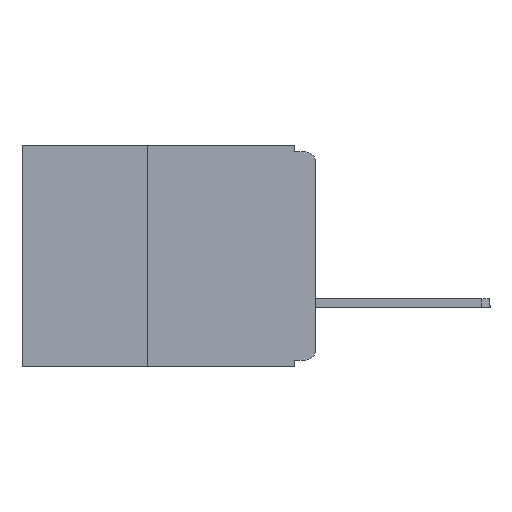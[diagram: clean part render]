
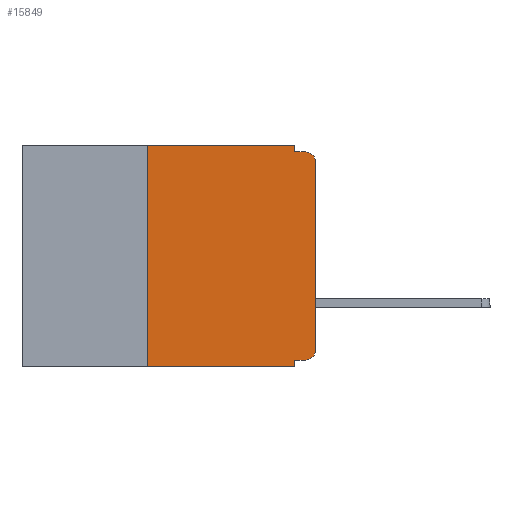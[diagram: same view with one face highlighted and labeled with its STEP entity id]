
A CAD part, left-side view. The second image highlights one B-rep face of the part: STEP entity #15849.
In plain terms, the highlighted planar face has unit normal (-1, 0, 0).
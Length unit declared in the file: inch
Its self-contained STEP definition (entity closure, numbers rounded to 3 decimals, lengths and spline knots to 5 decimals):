
#66 = DIRECTION ( 'NONE',  ( 0., -1., 0. ) ) ;
#398 = VERTEX_POINT ( 'NONE', #6209 ) ;
#481 = ORIENTED_EDGE ( 'NONE', *, *, #9868, .F. ) ;
#497 = CARTESIAN_POINT ( 'NONE',  ( 0., 0.031, -0.33 ) ) ;
#763 = VERTEX_POINT ( 'NONE', #16067 ) ;
#864 = VERTEX_POINT ( 'NONE', #1118 ) ;
#1118 = CARTESIAN_POINT ( 'NONE',  ( 0., 0.25, -0.33 ) ) ;
#1212 = CIRCLE ( 'NONE', #5402, 0.015 ) ;
#1240 = VECTOR ( 'NONE', #4410, 39.37008 ) ;
#1296 = FACE_OUTER_BOUND ( 'NONE', #16125, .T. ) ;
#1374 = EDGE_CURVE ( 'NONE', #15791, #12841, #13260, .T. ) ;
#1421 = AXIS2_PLACEMENT_3D ( 'NONE', #1442, #10555, #2855 ) ;
#1430 = EDGE_CURVE ( 'NONE', #864, #16133, #8579, .T. ) ;
#1442 = CARTESIAN_POINT ( 'NONE',  ( 0., 0.015, -0.305 ) ) ;
#1517 = EDGE_CURVE ( 'NONE', #864, #12063, #13790, .T. ) ;
#1592 = EDGE_CURVE ( 'NONE', #398, #12063, #15731, .T. ) ;
#1949 = VECTOR ( 'NONE', #4954, 39.37008 ) ;
#1961 = EDGE_CURVE ( 'NONE', #16133, #15791, #3544, .T. ) ;
#2298 = CIRCLE ( 'NONE', #1421, 0.015 ) ;
#2405 = CARTESIAN_POINT ( 'NONE',  ( 0., 0.437, 0. ) ) ;
#2565 = DIRECTION ( 'NONE',  ( 0., -1., 0. ) ) ;
#2602 = VECTOR ( 'NONE', #11193, 39.37008 ) ;
#2855 = DIRECTION ( 'NONE',  ( 0., 0., -1. ) ) ;
#3038 = ORIENTED_EDGE ( 'NONE', *, *, #10519, .T. ) ;
#3155 = VECTOR ( 'NONE', #2565, 39.37008 ) ;
#3258 = ORIENTED_EDGE ( 'NONE', *, *, #1517, .T. ) ;
#3544 = LINE ( 'NONE', #2405, #3155 ) ;
#3656 = ORIENTED_EDGE ( 'NONE', *, *, #1592, .F. ) ;
#4275 = ORIENTED_EDGE ( 'NONE', *, *, #9363, .F. ) ;
#4373 = CARTESIAN_POINT ( 'NONE',  ( 0., 0.031, 0. ) ) ;
#4410 = DIRECTION ( 'NONE',  ( 0., -1., 0. ) ) ;
#4485 = CARTESIAN_POINT ( 'NONE',  ( 0., 0.437, 0. ) ) ;
#4859 = LINE ( 'NONE', #8299, #1240 ) ;
#4954 = DIRECTION ( 'NONE',  ( 0., 0., 1. ) ) ;
#5307 = ORIENTED_EDGE ( 'NONE', *, *, #8946, .T. ) ;
#5323 = CARTESIAN_POINT ( 'NONE',  ( 0., 0., -0.32 ) ) ;
#5402 = AXIS2_PLACEMENT_3D ( 'NONE', #14794, #7637, #15915 ) ;
#5617 = AXIS2_PLACEMENT_3D ( 'NONE', #4485, #7090, #5811 ) ;
#5811 = DIRECTION ( 'NONE',  ( 0., 0., -1. ) ) ;
#6209 = CARTESIAN_POINT ( 'NONE',  ( 0., 0.031, -0.32 ) ) ;
#6341 = CARTESIAN_POINT ( 'NONE',  ( 0., 0., 0. ) ) ;
#6373 = ORIENTED_EDGE ( 'NONE', *, *, #1430, .F. ) ;
#7090 = DIRECTION ( 'NONE',  ( 1., 0., 0. ) ) ;
#7151 = VECTOR ( 'NONE', #13628, 39.37008 ) ;
#7637 = DIRECTION ( 'NONE',  ( -1., 0., 0. ) ) ;
#7971 = ORIENTED_EDGE ( 'NONE', *, *, #10731, .T. ) ;
#8163 = ORIENTED_EDGE ( 'NONE', *, *, #1374, .F. ) ;
#8299 = CARTESIAN_POINT ( 'NONE',  ( 0., 0., -0.01 ) ) ;
#8379 = VERTEX_POINT ( 'NONE', #12736 ) ;
#8503 = CARTESIAN_POINT ( 'NONE',  ( 0., 0.031, 0. ) ) ;
#8579 = LINE ( 'NONE', #13566, #1949 ) ;
#8634 = VERTEX_POINT ( 'NONE', #14252 ) ;
#8934 = ORIENTED_EDGE ( 'NONE', *, *, #1961, .F. ) ;
#8946 = EDGE_CURVE ( 'NONE', #8379, #9109, #10443, .T. ) ;
#9079 = LINE ( 'NONE', #5323, #15348 ) ;
#9109 = VERTEX_POINT ( 'NONE', #11525 ) ;
#9363 = EDGE_CURVE ( 'NONE', #12841, #8634, #4859, .T. ) ;
#9505 = CARTESIAN_POINT ( 'NONE',  ( 0., 0.437, -0.33 ) ) ;
#9709 = VECTOR ( 'NONE', #10794, 39.37008 ) ;
#9868 = EDGE_CURVE ( 'NONE', #763, #398, #9079, .T. ) ;
#9962 = CARTESIAN_POINT ( 'NONE',  ( 0., 0.031, -0.33 ) ) ;
#10443 = LINE ( 'NONE', #6341, #7151 ) ;
#10519 = EDGE_CURVE ( 'NONE', #9109, #8634, #1212, .T. ) ;
#10555 = DIRECTION ( 'NONE',  ( -1., 0., 0. ) ) ;
#10731 = EDGE_CURVE ( 'NONE', #763, #8379, #2298, .T. ) ;
#10794 = DIRECTION ( 'NONE',  ( 0., 0., -1. ) ) ;
#11193 = DIRECTION ( 'NONE',  ( 0., 0., -1. ) ) ;
#11525 = CARTESIAN_POINT ( 'NONE',  ( 0., 0., -0.025 ) ) ;
#12012 = PLANE ( 'NONE',  #5617 ) ;
#12063 = VERTEX_POINT ( 'NONE', #9962 ) ;
#12316 = CARTESIAN_POINT ( 'NONE',  ( 0., 0.25, 0. ) ) ;
#12736 = CARTESIAN_POINT ( 'NONE',  ( 0., 0., -0.305 ) ) ;
#12841 = VERTEX_POINT ( 'NONE', #13630 ) ;
#13260 = LINE ( 'NONE', #8503, #9709 ) ;
#13429 = VECTOR ( 'NONE', #66, 39.37008 ) ;
#13566 = CARTESIAN_POINT ( 'NONE',  ( 0., 0.25, -0.33 ) ) ;
#13628 = DIRECTION ( 'NONE',  ( 0., 0., 1. ) ) ;
#13630 = CARTESIAN_POINT ( 'NONE',  ( 0., 0.031, -0.01 ) ) ;
#13790 = LINE ( 'NONE', #9505, #13429 ) ;
#13913 = DIRECTION ( 'NONE',  ( 0., 1., 0. ) ) ;
#14252 = CARTESIAN_POINT ( 'NONE',  ( 0., 0.015, -0.01 ) ) ;
#14794 = CARTESIAN_POINT ( 'NONE',  ( 0., 0.015, -0.025 ) ) ;
#15348 = VECTOR ( 'NONE', #13913, 39.37008 ) ;
#15731 = LINE ( 'NONE', #497, #2602 ) ;
#15791 = VERTEX_POINT ( 'NONE', #4373 ) ;
#15849 = ADVANCED_FACE ( 'NONE', ( #1296 ), #12012, .F. ) ;
#15915 = DIRECTION ( 'NONE',  ( 0., 0., -1. ) ) ;
#16067 = CARTESIAN_POINT ( 'NONE',  ( 0., 0.015, -0.32 ) ) ;
#16125 = EDGE_LOOP ( 'NONE', ( #5307, #3038, #4275, #8163, #8934, #6373, #3258, #3656, #481, #7971 ) ) ;
#16133 = VERTEX_POINT ( 'NONE', #12316 ) ;
